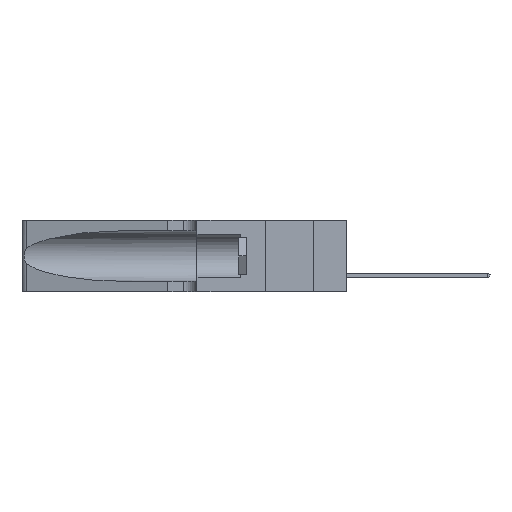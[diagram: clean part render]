
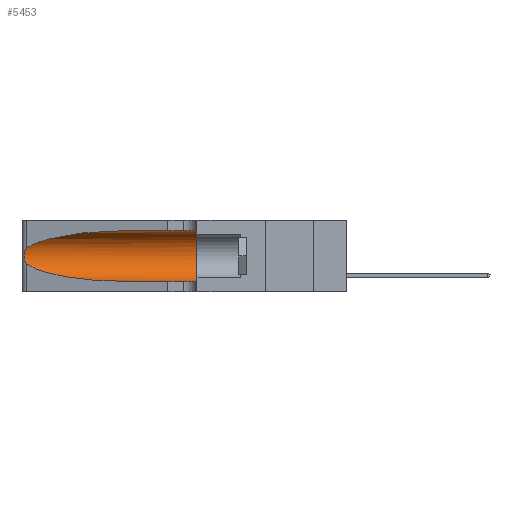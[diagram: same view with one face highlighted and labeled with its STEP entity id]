
A CAD part, left-side view. The second image highlights one B-rep face of the part: STEP entity #5453.
In plain terms, the highlighted cylindrical face has radius 3.308 mm (diameter 6.617 mm), a partial arc.
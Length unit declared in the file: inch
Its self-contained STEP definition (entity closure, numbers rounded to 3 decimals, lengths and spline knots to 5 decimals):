
#848 = AXIS2_PLACEMENT_3D ( 'NONE', #15844, #43714, #22980 ) ;
#1934 = EDGE_CURVE ( 'NONE', #41519, #6140, #3327, .T. ) ;
#3056 = CARTESIAN_POINT ( 'NONE',  ( 0.26075, 1.23896, 0.178 ) ) ;
#3184 = CARTESIAN_POINT ( 'NONE',  ( 0.2373, 1.15595, 0.28018 ) ) ;
#3327 = LINE ( 'NONE', #36885, #6585 ) ;
#3918 = EDGE_CURVE ( 'NONE', #9504, #15870, #6967, .T. ) ;
#5453 = ADVANCED_FACE ( 'NONE', ( #23920 ), #6587, .F. ) ;
#6140 = VERTEX_POINT ( 'NONE', #12978 ) ;
#6374 = CARTESIAN_POINT ( 'NONE',  ( 0.25639, 1.23184, 0.21858 ) ) ;
#6516 = CARTESIAN_POINT ( 'NONE',  ( 0.25856, 1.23593, 0.16098 ) ) ;
#6585 = VECTOR ( 'NONE', #16096, 39.37008 ) ;
#6587 = CYLINDRICAL_SURFACE ( 'NONE', #38188, 0.13025 ) ;
#6967 =( BOUNDED_CURVE ( )  B_SPLINE_CURVE ( 3, ( #21219, #7308, #10955, #13873 ),
 .UNSPECIFIED., .F., .F. ) 
 B_SPLINE_CURVE_WITH_KNOTS ( ( 4, 4 ),
 ( 3.44316, 4.71239 ),
 .UNSPECIFIED. ) 
 CURVE ( )  GEOMETRIC_REPRESENTATION_ITEM ( )  RATIONAL_B_SPLINE_CURVE ( ( 1., 0.87, 0.87, 1. ) ) 
 REPRESENTATION_ITEM ( '' )  );
#7308 = CARTESIAN_POINT ( 'NONE',  ( 0.2373, 1.15595, 0.08982 ) ) ;
#7326 = ORIENTED_EDGE ( 'NONE', *, *, #34323, .T. ) ;
#9302 = EDGE_CURVE ( 'NONE', #6140, #21178, #18618, .T. ) ;
#9504 = VERTEX_POINT ( 'NONE', #29677 ) ;
#9743 = CARTESIAN_POINT ( 'NONE',  ( 0.25487, 1.22718, 0.22369 ) ) ;
#9882 = CARTESIAN_POINT ( 'NONE',  ( 0.1305, 0.72297, 0.31525 ) ) ;
#10955 = CARTESIAN_POINT ( 'NONE',  ( 0.18966, 0.96281, 0.05475 ) ) ;
#11128 = B_SPLINE_CURVE_WITH_KNOTS ( 'NONE', 3,
 ( #30806, #40784, #6374, #16837, #41069, #20306, #23778, #3056, #27274, #6516, #37009, #38330, #24499, #27710 ),
 .UNSPECIFIED., .F., .F.,
 ( 4, 2, 2, 2, 2, 2, 4 ),
 ( 0., 0.00027, 0.00053, 0.00107, 0.0016, 0.00187, 0.00214 ),
 .UNSPECIFIED. ) ;
#12978 = CARTESIAN_POINT ( 'NONE',  ( 0.1305, 0.35, 0.31525 ) ) ;
#13873 = CARTESIAN_POINT ( 'NONE',  ( 0.1305, 0.72297, 0.05475 ) ) ;
#14349 = EDGE_CURVE ( 'NONE', #34074, #9504, #11128, .T. ) ;
#14648 = VECTOR ( 'NONE', #21375, 39.37008 ) ;
#14829 = CARTESIAN_POINT ( 'NONE',  ( 0.1305, 0.72297, 0.31525 ) ) ;
#15844 = CARTESIAN_POINT ( 'NONE',  ( 0.1305, 0.35, 0.185 ) ) ;
#15870 = VERTEX_POINT ( 'NONE', #23713 ) ;
#16096 = DIRECTION ( 'NONE',  ( 0., -1., 0. ) ) ;
#16837 = CARTESIAN_POINT ( 'NONE',  ( 0.25787, 1.23484, 0.2124 ) ) ;
#18618 = CIRCLE ( 'NONE', #848, 0.13025 ) ;
#20306 = CARTESIAN_POINT ( 'NONE',  ( 0.26018, 1.23835, 0.19895 ) ) ;
#21178 = VERTEX_POINT ( 'NONE', #28223 ) ;
#21219 = CARTESIAN_POINT ( 'NONE',  ( 0.25487, 1.22718, 0.14631 ) ) ;
#21375 = DIRECTION ( 'NONE',  ( 0., -1., 0. ) ) ;
#22980 = DIRECTION ( 'NONE',  ( 0., 0., 1. ) ) ;
#23713 = CARTESIAN_POINT ( 'NONE',  ( 0.1305, 0.72297, 0.05475 ) ) ;
#23778 = CARTESIAN_POINT ( 'NONE',  ( 0.26075, 1.23896, 0.19203 ) ) ;
#23920 = FACE_OUTER_BOUND ( 'NONE', #41911, .T. ) ;
#23996 = ORIENTED_EDGE ( 'NONE', *, *, #14349, .T. ) ;
#24499 = CARTESIAN_POINT ( 'NONE',  ( 0.25555, 1.22993, 0.14849 ) ) ;
#26345 = ORIENTED_EDGE ( 'NONE', *, *, #32036, .T. ) ;
#27274 = CARTESIAN_POINT ( 'NONE',  ( 0.26017, 1.23833, 0.17102 ) ) ;
#27710 = CARTESIAN_POINT ( 'NONE',  ( 0.25487, 1.22718, 0.14631 ) ) ;
#28223 = CARTESIAN_POINT ( 'NONE',  ( 0.1305, 0.35, 0.05475 ) ) ;
#29677 = CARTESIAN_POINT ( 'NONE',  ( 0.25487, 1.22718, 0.14631 ) ) ;
#30806 = CARTESIAN_POINT ( 'NONE',  ( 0.25487, 1.22718, 0.22369 ) ) ;
#30969 = CARTESIAN_POINT ( 'NONE',  ( 0.1305, 1.61858, 0.185 ) ) ;
#31807 = DIRECTION ( 'NONE',  ( 0., 0., -1. ) ) ;
#32036 = EDGE_CURVE ( 'NONE', #15870, #21178, #43433, .T. ) ;
#32326 = CARTESIAN_POINT ( 'NONE',  ( 0.1305, 1.61858, 0.05475 ) ) ;
#33994 = CARTESIAN_POINT ( 'NONE',  ( 0.18966, 0.96281, 0.31525 ) ) ;
#34074 = VERTEX_POINT ( 'NONE', #36733 ) ;
#34185 = ORIENTED_EDGE ( 'NONE', *, *, #9302, .F. ) ;
#34323 = EDGE_CURVE ( 'NONE', #41519, #34074, #36724, .T. ) ;
#36724 =( BOUNDED_CURVE ( )  B_SPLINE_CURVE ( 3, ( #9882, #33994, #3184, #9743 ),
 .UNSPECIFIED., .F., .T. ) 
 B_SPLINE_CURVE_WITH_KNOTS ( ( 4, 4 ),
 ( 1.5708, 2.84003 ),
 .UNSPECIFIED. ) 
 CURVE ( )  GEOMETRIC_REPRESENTATION_ITEM ( )  RATIONAL_B_SPLINE_CURVE ( ( 1., 0.87, 0.87, 1. ) ) 
 REPRESENTATION_ITEM ( '' )  );
#36733 = CARTESIAN_POINT ( 'NONE',  ( 0.25487, 1.22718, 0.22369 ) ) ;
#36885 = CARTESIAN_POINT ( 'NONE',  ( 0.1305, 1.61858, 0.31525 ) ) ;
#37009 = CARTESIAN_POINT ( 'NONE',  ( 0.25789, 1.23486, 0.15765 ) ) ;
#38188 = AXIS2_PLACEMENT_3D ( 'NONE', #30969, #39377, #31807 ) ;
#38330 = CARTESIAN_POINT ( 'NONE',  ( 0.25639, 1.23186, 0.15144 ) ) ;
#39377 = DIRECTION ( 'NONE',  ( 0., -1., 0. ) ) ;
#39683 = ORIENTED_EDGE ( 'NONE', *, *, #3918, .T. ) ;
#40784 = CARTESIAN_POINT ( 'NONE',  ( 0.25555, 1.22994, 0.2215 ) ) ;
#41069 = CARTESIAN_POINT ( 'NONE',  ( 0.25854, 1.2359, 0.20912 ) ) ;
#41519 = VERTEX_POINT ( 'NONE', #14829 ) ;
#41911 = EDGE_LOOP ( 'NONE', ( #7326, #23996, #39683, #26345, #34185, #42781 ) ) ;
#42781 = ORIENTED_EDGE ( 'NONE', *, *, #1934, .F. ) ;
#43433 = LINE ( 'NONE', #32326, #14648 ) ;
#43714 = DIRECTION ( 'NONE',  ( 0., 1., 0. ) ) ;
